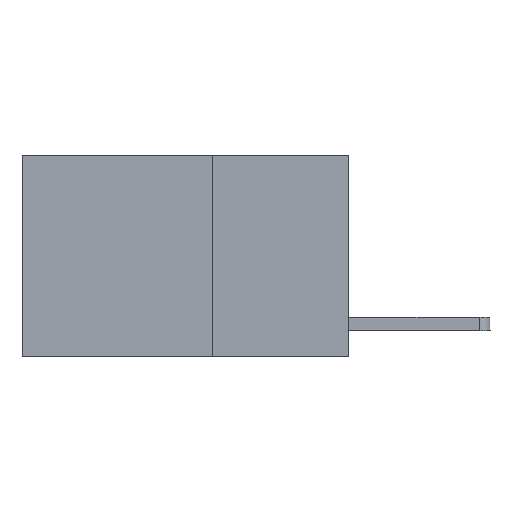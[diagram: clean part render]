
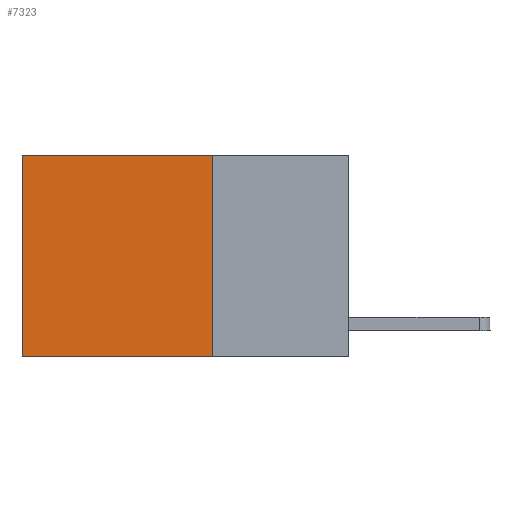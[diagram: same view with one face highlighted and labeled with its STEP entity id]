
A CAD part, left-side view. The second image highlights one B-rep face of the part: STEP entity #7323.
In plain terms, the highlighted planar face has unit normal (-1, 0, 0).
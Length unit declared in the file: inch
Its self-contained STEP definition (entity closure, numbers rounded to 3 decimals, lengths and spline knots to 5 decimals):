
#300 = ORIENTED_EDGE ( 'NONE', *, *, #8983, .F. ) ;
#404 = LINE ( 'NONE', #8710, #8187 ) ;
#510 = CARTESIAN_POINT ( 'NONE',  ( 0.2625, 0.6, -0.37 ) ) ;
#782 = VECTOR ( 'NONE', #4774, 39.37008 ) ;
#825 = LINE ( 'NONE', #1708, #9183 ) ;
#906 = FACE_OUTER_BOUND ( 'NONE', #3072, .T. ) ;
#1018 = LINE ( 'NONE', #1622, #1455 ) ;
#1455 = VECTOR ( 'NONE', #7352, 39.37008 ) ;
#1622 = CARTESIAN_POINT ( 'NONE',  ( 0.2625, 0.6, 0. ) ) ;
#1708 = CARTESIAN_POINT ( 'NONE',  ( 0.2625, 0.25, -0.37 ) ) ;
#1789 = CARTESIAN_POINT ( 'NONE',  ( 0.2625, 0.25, 0. ) ) ;
#2351 = DIRECTION ( 'NONE',  ( 1., 0., 0. ) ) ;
#2568 = ORIENTED_EDGE ( 'NONE', *, *, #3931, .T. ) ;
#3072 = EDGE_LOOP ( 'NONE', ( #2568, #5517, #300, #7387 ) ) ;
#3094 = CARTESIAN_POINT ( 'NONE',  ( 0.2625, 0.25, 0. ) ) ;
#3242 = CARTESIAN_POINT ( 'NONE',  ( 0.2625, 0.25, 0. ) ) ;
#3254 = DIRECTION ( 'NONE',  ( 0., 0., -1. ) ) ;
#3774 = AXIS2_PLACEMENT_3D ( 'NONE', #3094, #2351, #5840 ) ;
#3931 = EDGE_CURVE ( 'NONE', #4233, #6797, #1018, .T. ) ;
#4233 = VERTEX_POINT ( 'NONE', #6414 ) ;
#4504 = VERTEX_POINT ( 'NONE', #3242 ) ;
#4774 = DIRECTION ( 'NONE',  ( 0., 1., 0. ) ) ;
#5517 = ORIENTED_EDGE ( 'NONE', *, *, #5608, .F. ) ;
#5608 = EDGE_CURVE ( 'NONE', #6112, #6797, #825, .T. ) ;
#5840 = DIRECTION ( 'NONE',  ( 0., 0., -1. ) ) ;
#6112 = VERTEX_POINT ( 'NONE', #7902 ) ;
#6414 = CARTESIAN_POINT ( 'NONE',  ( 0.2625, 0.6, 0. ) ) ;
#6496 = PLANE ( 'NONE',  #3774 ) ;
#6797 = VERTEX_POINT ( 'NONE', #510 ) ;
#7254 = DIRECTION ( 'NONE',  ( 0., 1., 0. ) ) ;
#7323 = ADVANCED_FACE ( 'NONE', ( #906 ), #6496, .F. ) ;
#7352 = DIRECTION ( 'NONE',  ( 0., 0., -1. ) ) ;
#7387 = ORIENTED_EDGE ( 'NONE', *, *, #7505, .T. ) ;
#7474 = LINE ( 'NONE', #1789, #782 ) ;
#7505 = EDGE_CURVE ( 'NONE', #4504, #4233, #7474, .T. ) ;
#7902 = CARTESIAN_POINT ( 'NONE',  ( 0.2625, 0.25, -0.37 ) ) ;
#8187 = VECTOR ( 'NONE', #3254, 39.37008 ) ;
#8710 = CARTESIAN_POINT ( 'NONE',  ( 0.2625, 0.25, 0. ) ) ;
#8983 = EDGE_CURVE ( 'NONE', #4504, #6112, #404, .T. ) ;
#9183 = VECTOR ( 'NONE', #7254, 39.37008 ) ;
